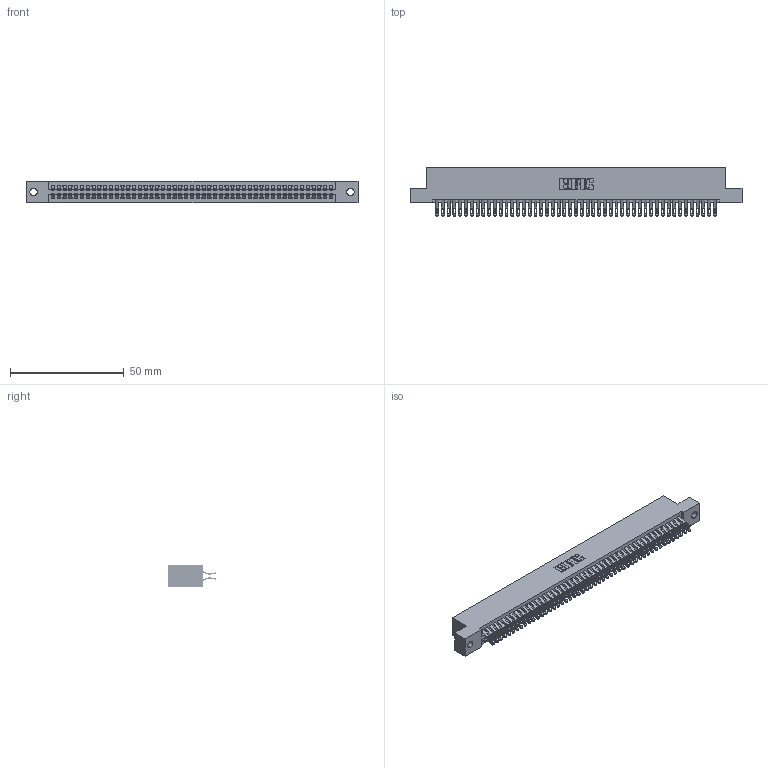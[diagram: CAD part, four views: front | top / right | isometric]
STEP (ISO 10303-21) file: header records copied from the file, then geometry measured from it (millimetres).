
FILE_DESCRIPTION (( 'STEP AP203' ), '1' );
FILE_NAME ('395-098-555-202.STEP', '2019-10-26T13:40:31', ( '' ), ( '' ), 'SwSTEP 2.0', 'SolidWorks 2016', '' );
FILE_SCHEMA (( 'CONFIG_CONTROL_DESIGN' ));
Length unit declared in the file: inch
Products named in the file (3): 395-098-555-202; 345 Part_Flush Mounting Lugs - 0.128 Dia; 345-292-001_555 Tail
Assembly tree (99 placements, depth 2):
  395-098-555-202
    345 Part_Flush Mounting Lugs - 0.128 Dia
    345-292-001_555 Tail  x98
Bounding box: 145.67 x 21.13 x 9.4 mm (x, y, z)
Volume: 14463 mm3; surface area: 22230.2 mm2
Topology: 99 solids, 99 shells, 5614 faces, 17687 edges, 11790 vertices
Faces by surface type: plane 3118, cylinder 2496
Entity records: 37833 total; most frequent: CARTESIAN_POINT 6370, ORIENTED_EDGE 6274, DIRECTION 5577, EDGE_CURVE 3137, LINE 2789, VECTOR 2789, VERTEX_POINT 2090, AXIS2_PLACEMENT_3D 1394
